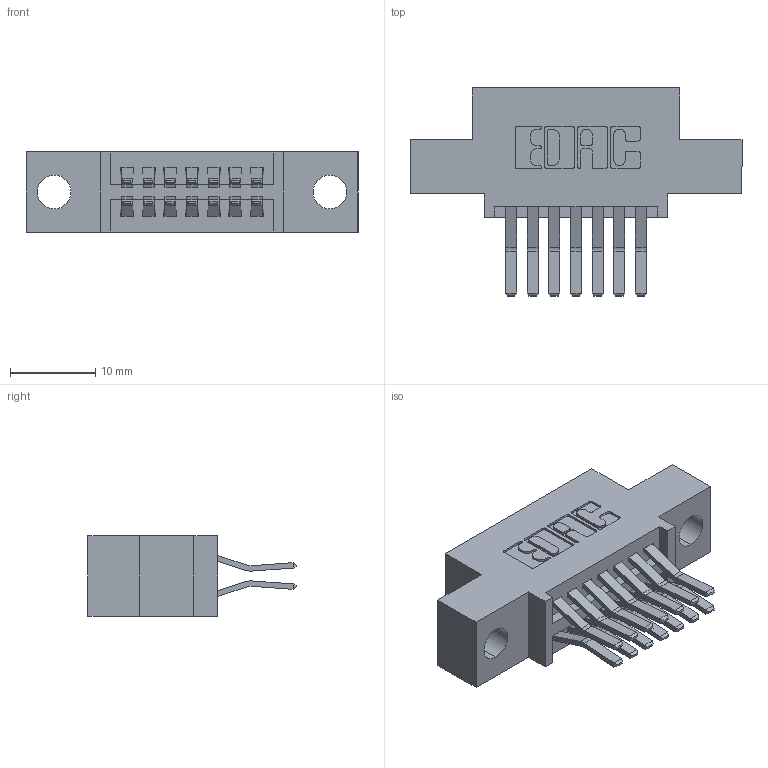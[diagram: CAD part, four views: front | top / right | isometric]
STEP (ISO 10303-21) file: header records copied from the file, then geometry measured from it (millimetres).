
FILE_DESCRIPTION (( 'STEP AP203' ), '1' );
FILE_NAME ('345-014-560-504.STEP', '2018-08-18T18:57:22', ( '' ), ( '' ), 'SwSTEP 2.0', 'SolidWorks 2016', '' );
FILE_SCHEMA (( 'CONFIG_CONTROL_DESIGN' ));
Length unit declared in the file: inch
Products named in the file (3): 345 Part_0.110 Offset - 0.156 Dia-TH; 345-292-001_560 Tail; 345-014-560-504
Assembly tree (15 placements, depth 2):
  345-014-560-504
    345 Part_0.110 Offset - 0.156 Dia-TH
    345-292-001_560 Tail  x14
Bounding box: 38.99 x 24.45 x 9.4 mm (x, y, z)
Volume: 3393.1 mm3; surface area: 4481.7 mm2
Topology: 15 solids, 15 shells, 858 faces, 2523 edges, 1662 vertices
Faces by surface type: plane 546, cylinder 312
Entity records: 10427 total; most frequent: CARTESIAN_POINT 1784, ORIENTED_EDGE 1718, DIRECTION 1619, EDGE_CURVE 859, VECTOR 695, LINE 695, VERTEX_POINT 570, AXIS2_PLACEMENT_3D 462
